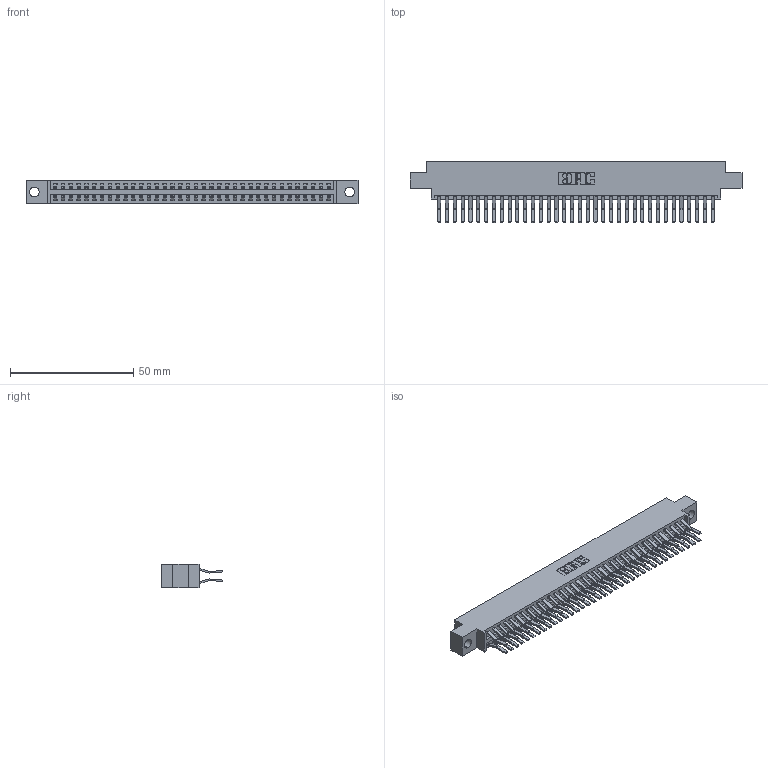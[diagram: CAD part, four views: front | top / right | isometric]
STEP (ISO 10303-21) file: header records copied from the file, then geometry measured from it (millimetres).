
FILE_DESCRIPTION (( 'STEP AP203' ), '1' );
FILE_NAME ('346-072-560-804.STEP', '2022-05-25T01:17:24', ( '' ), ( '' ), 'SwSTEP 2.0', 'SolidWorks 2020', '' );
FILE_SCHEMA (( 'CONFIG_CONTROL_DESIGN' ));
Length unit declared in the file: inch
Products named in the file (3): 346 Part_0.170 Offset - 0.156 Dia-TH; 345-292-001_560 Tail; 346-072-560-804
Assembly tree (73 placements, depth 2):
  346-072-560-804
    346 Part_0.170 Offset - 0.156 Dia-TH
    345-292-001_560 Tail  x72
Bounding box: 134.87 x 24.78 x 9.4 mm (x, y, z)
Volume: 13316.7 mm3; surface area: 19496.9 mm2
Topology: 73 solids, 73 shells, 4028 faces, 11969 edges, 7882 vertices
Faces by surface type: plane 2614, cylinder 1414
Entity records: 24941 total; most frequent: CARTESIAN_POINT 4126, ORIENTED_EDGE 4058, DIRECTION 3689, EDGE_CURVE 2029, LINE 1749, VECTOR 1749, VERTEX_POINT 1350, AXIS2_PLACEMENT_3D 970
